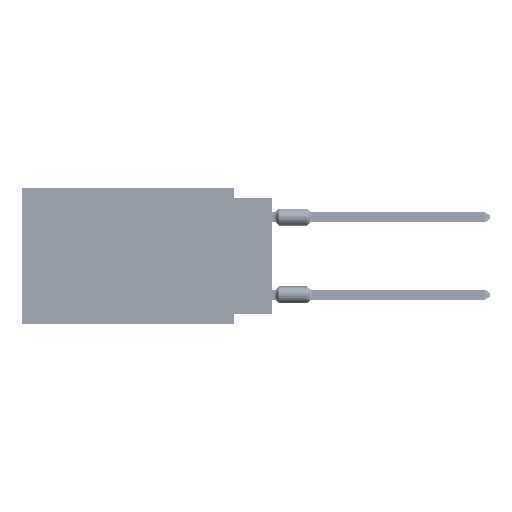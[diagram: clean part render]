
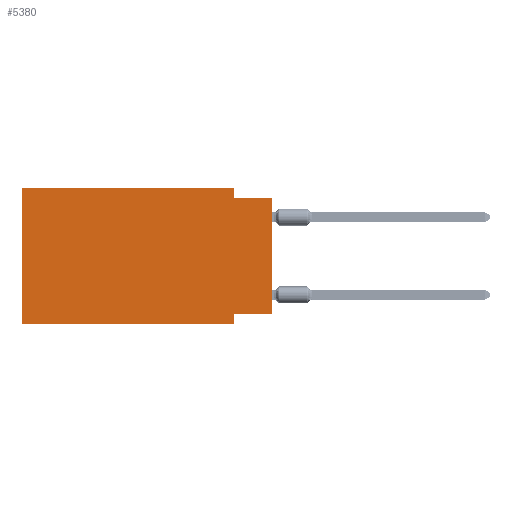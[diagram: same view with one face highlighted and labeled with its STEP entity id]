
A CAD part, left-side view. The second image highlights one B-rep face of the part: STEP entity #5380.
In plain terms, the highlighted planar face has unit normal (-1, 0, 0).
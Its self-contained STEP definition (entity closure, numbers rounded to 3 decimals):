
#1277 = EDGE_CURVE ( 'NONE', #43323, #85510, #55604, .T. ) ;
#5380 = ADVANCED_FACE ( 'NONE', ( #97917 ), #98476, .F. ) ;
#9003 = EDGE_CURVE ( 'NONE', #47708, #113649, #100512, .T. ) ;
#9357 = CARTESIAN_POINT ( 'NONE',  ( 0., 0., -0.635 ) ) ;
#9635 = DIRECTION ( 'NONE',  ( 0., 0., -1. ) ) ;
#11377 = ORIENTED_EDGE ( 'NONE', *, *, #63289, .F. ) ;
#12545 = VERTEX_POINT ( 'NONE', #52429 ) ;
#14138 = LINE ( 'NONE', #49753, #33107 ) ;
#15025 = LINE ( 'NONE', #89038, #25854 ) ;
#18493 = CARTESIAN_POINT ( 'NONE',  ( 0., 16.383, 0. ) ) ;
#19533 = VECTOR ( 'NONE', #112617, 1000. ) ;
#19765 = CARTESIAN_POINT ( 'NONE',  ( 0., 2.54, -0.635 ) ) ;
#20616 = VERTEX_POINT ( 'NONE', #36388 ) ;
#24952 = ORIENTED_EDGE ( 'NONE', *, *, #43437, .F. ) ;
#25462 = DIRECTION ( 'NONE',  ( 1., 0., 0. ) ) ;
#25854 = VECTOR ( 'NONE', #106029, 1000. ) ;
#25954 = CARTESIAN_POINT ( 'NONE',  ( 0., 16.383, -8.89 ) ) ;
#26125 = LINE ( 'NONE', #18493, #36055 ) ;
#26450 = ORIENTED_EDGE ( 'NONE', *, *, #9003, .F. ) ;
#29761 = AXIS2_PLACEMENT_3D ( 'NONE', #89692, #25462, #9635 ) ;
#31576 = LINE ( 'NONE', #77121, #91414 ) ;
#33107 = VECTOR ( 'NONE', #76625, 1000. ) ;
#33386 = CARTESIAN_POINT ( 'NONE',  ( 0., 2.54, -8.89 ) ) ;
#35892 = CARTESIAN_POINT ( 'NONE',  ( 0., 0., -8.255 ) ) ;
#36055 = VECTOR ( 'NONE', #108481, 1000. ) ;
#36388 = CARTESIAN_POINT ( 'NONE',  ( 0., 2.54, -8.255 ) ) ;
#39601 = VECTOR ( 'NONE', #47311, 1000. ) ;
#40910 = LINE ( 'NONE', #77693, #112460 ) ;
#43323 = VERTEX_POINT ( 'NONE', #25954 ) ;
#43437 = EDGE_CURVE ( 'NONE', #12545, #47708, #15025, .T. ) ;
#45229 = VERTEX_POINT ( 'NONE', #35892 ) ;
#45287 = EDGE_CURVE ( 'NONE', #106891, #12545, #31576, .T. ) ;
#47311 = DIRECTION ( 'NONE',  ( 0., -1., 0. ) ) ;
#47708 = VERTEX_POINT ( 'NONE', #19765 ) ;
#48010 = DIRECTION ( 'NONE',  ( 0., -1., 0. ) ) ;
#49351 = EDGE_CURVE ( 'NONE', #43323, #106891, #26125, .T. ) ;
#49484 = CARTESIAN_POINT ( 'NONE',  ( 0., 2.54, -8.89 ) ) ;
#49753 = CARTESIAN_POINT ( 'NONE',  ( 0., 0., -8.255 ) ) ;
#50621 = LINE ( 'NONE', #49484, #19533 ) ;
#52429 = CARTESIAN_POINT ( 'NONE',  ( 0., 2.54, 0. ) ) ;
#55604 = LINE ( 'NONE', #101814, #79460 ) ;
#55777 = ORIENTED_EDGE ( 'NONE', *, *, #45287, .F. ) ;
#60137 = DIRECTION ( 'NONE',  ( 0., 0., 1. ) ) ;
#63289 = EDGE_CURVE ( 'NONE', #45229, #20616, #14138, .T. ) ;
#64465 = DIRECTION ( 'NONE',  ( 0., -1., 0. ) ) ;
#67271 = ORIENTED_EDGE ( 'NONE', *, *, #49351, .F. ) ;
#72308 = ORIENTED_EDGE ( 'NONE', *, *, #1277, .T. ) ;
#72914 = ORIENTED_EDGE ( 'NONE', *, *, #75796, .F. ) ;
#75796 = EDGE_CURVE ( 'NONE', #20616, #85510, #50621, .T. ) ;
#76625 = DIRECTION ( 'NONE',  ( 0., 1., 0. ) ) ;
#77024 = CARTESIAN_POINT ( 'NONE',  ( 0., 0., -0.635 ) ) ;
#77121 = CARTESIAN_POINT ( 'NONE',  ( 0., 16.383, 0. ) ) ;
#77693 = CARTESIAN_POINT ( 'NONE',  ( 0., 0., 0. ) ) ;
#79460 = VECTOR ( 'NONE', #48010, 1000. ) ;
#85510 = VERTEX_POINT ( 'NONE', #33386 ) ;
#89038 = CARTESIAN_POINT ( 'NONE',  ( 0., 2.54, 0. ) ) ;
#89245 = ORIENTED_EDGE ( 'NONE', *, *, #91608, .T. ) ;
#89692 = CARTESIAN_POINT ( 'NONE',  ( 0., 16.383, 0. ) ) ;
#90483 = EDGE_LOOP ( 'NONE', ( #89245, #26450, #24952, #55777, #67271, #72308, #72914, #11377 ) ) ;
#91414 = VECTOR ( 'NONE', #64465, 1000. ) ;
#91608 = EDGE_CURVE ( 'NONE', #45229, #113649, #40910, .T. ) ;
#97917 = FACE_OUTER_BOUND ( 'NONE', #90483, .T. ) ;
#98476 = PLANE ( 'NONE',  #29761 ) ;
#100512 = LINE ( 'NONE', #9357, #39601 ) ;
#101814 = CARTESIAN_POINT ( 'NONE',  ( 0., 16.383, -8.89 ) ) ;
#106029 = DIRECTION ( 'NONE',  ( 0., 0., -1. ) ) ;
#106825 = CARTESIAN_POINT ( 'NONE',  ( 0., 16.383, 0. ) ) ;
#106891 = VERTEX_POINT ( 'NONE', #106825 ) ;
#108481 = DIRECTION ( 'NONE',  ( 0., 0., 1. ) ) ;
#112460 = VECTOR ( 'NONE', #60137, 1000. ) ;
#112617 = DIRECTION ( 'NONE',  ( 0., 0., -1. ) ) ;
#113649 = VERTEX_POINT ( 'NONE', #77024 ) ;
